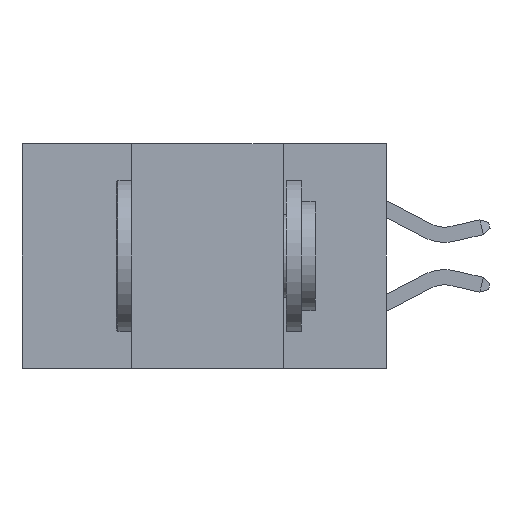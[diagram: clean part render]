
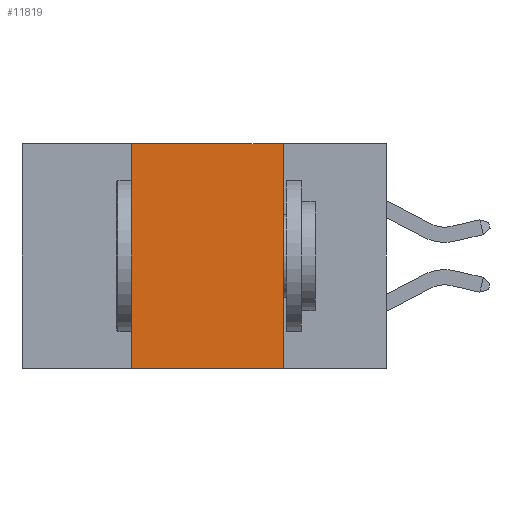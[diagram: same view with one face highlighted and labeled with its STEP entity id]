
A CAD part, left-side view. The second image highlights one B-rep face of the part: STEP entity #11819.
In plain terms, the highlighted planar face has unit normal (-1, 0, 0).
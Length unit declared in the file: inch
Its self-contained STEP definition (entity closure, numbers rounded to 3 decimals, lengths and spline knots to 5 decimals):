
#40 = CARTESIAN_POINT ( 'NONE',  ( 0., 0.6, 0. ) ) ;
#220 = VECTOR ( 'NONE', #11012, 39.37008 ) ;
#747 = ORIENTED_EDGE ( 'NONE', *, *, #11849, .F. ) ;
#1454 = CARTESIAN_POINT ( 'NONE',  ( 0., 0.6, -0.37 ) ) ;
#1681 = DIRECTION ( 'NONE',  ( 0., 0., -1. ) ) ;
#1749 = FACE_OUTER_BOUND ( 'NONE', #3808, .T. ) ;
#2977 = CARTESIAN_POINT ( 'NONE',  ( 0., 0.17, -0.37 ) ) ;
#3049 = ORIENTED_EDGE ( 'NONE', *, *, #8686, .T. ) ;
#3682 = CARTESIAN_POINT ( 'NONE',  ( 0., 0.42, -0.37 ) ) ;
#3763 = AXIS2_PLACEMENT_3D ( 'NONE', #10480, #5415, #1681 ) ;
#3808 = EDGE_LOOP ( 'NONE', ( #747, #5781, #12569, #3049 ) ) ;
#3917 = VECTOR ( 'NONE', #6071, 39.37008 ) ;
#4560 = VERTEX_POINT ( 'NONE', #2977 ) ;
#5031 = EDGE_CURVE ( 'NONE', #9992, #8030, #11715, .T. ) ;
#5415 = DIRECTION ( 'NONE',  ( 1., 0., 0. ) ) ;
#5781 = ORIENTED_EDGE ( 'NONE', *, *, #5031, .F. ) ;
#6071 = DIRECTION ( 'NONE',  ( 0., 0., 1. ) ) ;
#6198 = LINE ( 'NONE', #11896, #3917 ) ;
#6463 = CARTESIAN_POINT ( 'NONE',  ( 0., 0.42, 0. ) ) ;
#7759 = DIRECTION ( 'NONE',  ( 0., -1., 0. ) ) ;
#8030 = VERTEX_POINT ( 'NONE', #11567 ) ;
#8340 = PLANE ( 'NONE',  #3763 ) ;
#8401 = DIRECTION ( 'NONE',  ( 0., 0., -1. ) ) ;
#8686 = EDGE_CURVE ( 'NONE', #9682, #4560, #10233, .T. ) ;
#9080 = VECTOR ( 'NONE', #7759, 39.37008 ) ;
#9215 = EDGE_CURVE ( 'NONE', #9682, #9992, #6198, .T. ) ;
#9682 = VERTEX_POINT ( 'NONE', #3682 ) ;
#9992 = VERTEX_POINT ( 'NONE', #6463 ) ;
#10233 = LINE ( 'NONE', #1454, #220 ) ;
#10480 = CARTESIAN_POINT ( 'NONE',  ( 0., 0.6, 0. ) ) ;
#11012 = DIRECTION ( 'NONE',  ( 0., -1., 0. ) ) ;
#11155 = VECTOR ( 'NONE', #8401, 39.37008 ) ;
#11567 = CARTESIAN_POINT ( 'NONE',  ( 0., 0.17, 0. ) ) ;
#11715 = LINE ( 'NONE', #40, #9080 ) ;
#11819 = ADVANCED_FACE ( 'NONE', ( #1749 ), #8340, .F. ) ;
#11849 = EDGE_CURVE ( 'NONE', #8030, #4560, #12500, .T. ) ;
#11896 = CARTESIAN_POINT ( 'NONE',  ( 0., 0.42, -0.37 ) ) ;
#12261 = CARTESIAN_POINT ( 'NONE',  ( 0., 0.17, -0.37 ) ) ;
#12500 = LINE ( 'NONE', #12261, #11155 ) ;
#12569 = ORIENTED_EDGE ( 'NONE', *, *, #9215, .F. ) ;
